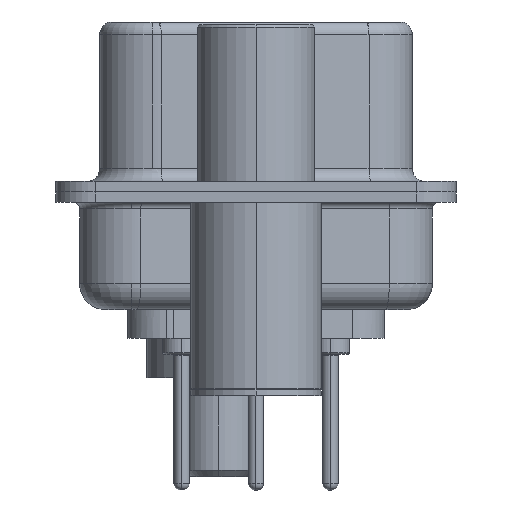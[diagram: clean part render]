
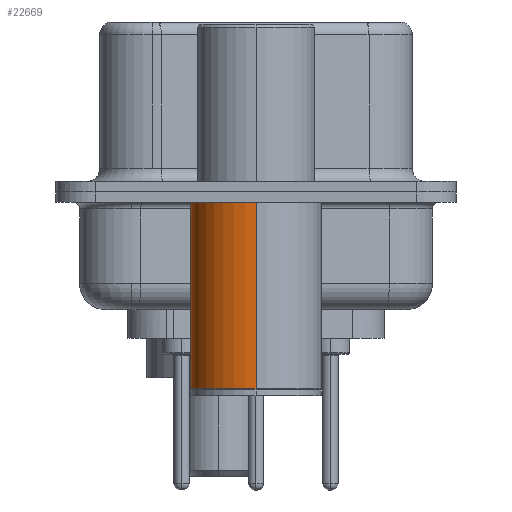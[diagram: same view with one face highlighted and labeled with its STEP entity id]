
A CAD part, left-side view. The second image highlights one B-rep face of the part: STEP entity #22669.
In plain terms, the highlighted cylindrical face has radius 2.5 mm (diameter 5 mm), a partial arc.
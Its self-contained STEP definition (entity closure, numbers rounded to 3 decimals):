
#843 = ORIENTED_EDGE ( 'NONE', *, *, #13914, .F. ) ;
#2000 = FACE_OUTER_BOUND ( 'NONE', #26886, .T. ) ;
#3727 = CARTESIAN_POINT ( 'NONE',  ( 2.5, 0., -7.525 ) ) ;
#3931 = VECTOR ( 'NONE', #15191, 1000. ) ;
#4225 = EDGE_CURVE ( 'NONE', #29745, #16663, #10707, .T. ) ;
#4281 = AXIS2_PLACEMENT_3D ( 'NONE', #26130, #26066, #26888 ) ;
#4871 = VERTEX_POINT ( 'NONE', #3727 ) ;
#5777 = CARTESIAN_POINT ( 'NONE',  ( 0., 0., -7.525 ) ) ;
#6830 = CYLINDRICAL_SURFACE ( 'NONE', #15707, 2.5 ) ;
#7773 = ORIENTED_EDGE ( 'NONE', *, *, #18364, .T. ) ;
#8180 = DIRECTION ( 'NONE',  ( 1., 0., 0. ) ) ;
#9691 = CARTESIAN_POINT ( 'NONE',  ( 2.5, 0., -0.4 ) ) ;
#10707 = CIRCLE ( 'NONE', #4281, 2.5 ) ;
#12848 = CARTESIAN_POINT ( 'NONE',  ( 2.5, 0., 0.581 ) ) ;
#13803 = AXIS2_PLACEMENT_3D ( 'NONE', #5777, #22075, #8180 ) ;
#13914 = EDGE_CURVE ( 'NONE', #4871, #29745, #16454, .T. ) ;
#13942 = CIRCLE ( 'NONE', #13803, 2.5 ) ;
#15191 = DIRECTION ( 'NONE',  ( 0., 0., 1. ) ) ;
#15707 = AXIS2_PLACEMENT_3D ( 'NONE', #18615, #16331, #23142 ) ;
#16058 = EDGE_CURVE ( 'NONE', #4871, #29057, #13942, .T. ) ;
#16331 = DIRECTION ( 'NONE',  ( 0., 0., 1. ) ) ;
#16454 = LINE ( 'NONE', #12848, #3931 ) ;
#16530 = ORIENTED_EDGE ( 'NONE', *, *, #16058, .T. ) ;
#16663 = VERTEX_POINT ( 'NONE', #23568 ) ;
#17786 = VECTOR ( 'NONE', #23268, 1000. ) ;
#18364 = EDGE_CURVE ( 'NONE', #29057, #16663, #24592, .T. ) ;
#18615 = CARTESIAN_POINT ( 'NONE',  ( 0., 0., 0.581 ) ) ;
#18953 = CARTESIAN_POINT ( 'NONE',  ( -2.5, 0., -7.525 ) ) ;
#20993 = CARTESIAN_POINT ( 'NONE',  ( -2.5, 0., 0.581 ) ) ;
#22075 = DIRECTION ( 'NONE',  ( 0., 0., 1. ) ) ;
#22669 = ADVANCED_FACE ( 'NONE', ( #2000 ), #6830, .T. ) ;
#23142 = DIRECTION ( 'NONE',  ( 1., 0., 0. ) ) ;
#23268 = DIRECTION ( 'NONE',  ( 0., 0., 1. ) ) ;
#23568 = CARTESIAN_POINT ( 'NONE',  ( -2.5, 0., -0.4 ) ) ;
#24592 = LINE ( 'NONE', #20993, #17786 ) ;
#24965 = ORIENTED_EDGE ( 'NONE', *, *, #4225, .F. ) ;
#26066 = DIRECTION ( 'NONE',  ( 0., 0., 1. ) ) ;
#26130 = CARTESIAN_POINT ( 'NONE',  ( 0., 0., -0.4 ) ) ;
#26886 = EDGE_LOOP ( 'NONE', ( #16530, #7773, #24965, #843 ) ) ;
#26888 = DIRECTION ( 'NONE',  ( 1., 0., 0. ) ) ;
#29057 = VERTEX_POINT ( 'NONE', #18953 ) ;
#29745 = VERTEX_POINT ( 'NONE', #9691 ) ;
